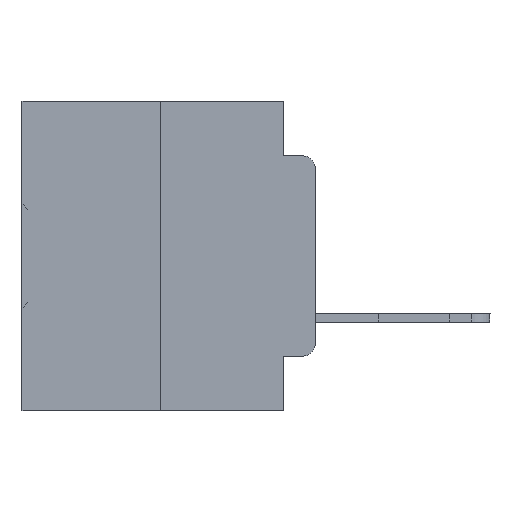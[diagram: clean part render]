
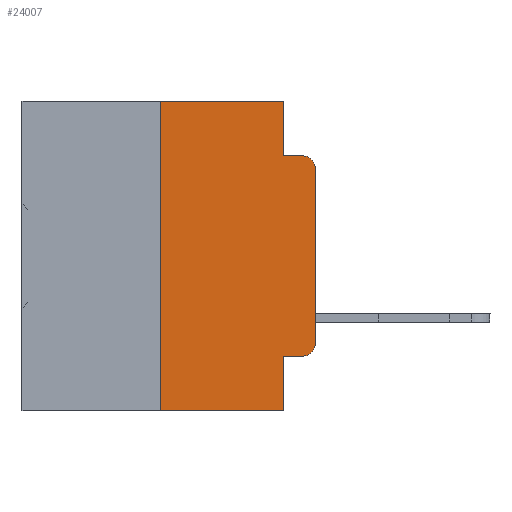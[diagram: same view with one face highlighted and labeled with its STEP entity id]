
A CAD part, left-side view. The second image highlights one B-rep face of the part: STEP entity #24007.
In plain terms, the highlighted planar face has unit normal (-1, 0, 0).
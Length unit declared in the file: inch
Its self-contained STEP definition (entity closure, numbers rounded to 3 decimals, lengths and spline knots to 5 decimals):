
#1431 = DIRECTION ( 'NONE',  ( 0., -1., 0. ) ) ;
#1639 = CARTESIAN_POINT ( 'NONE',  ( 0., 0.02, -0.3915 ) ) ;
#1751 = EDGE_CURVE ( 'NONE', #10572, #32576, #12706, .T. ) ;
#2280 = DIRECTION ( 'NONE',  ( 0., 0., -1. ) ) ;
#2330 = CARTESIAN_POINT ( 'NONE',  ( 0., 0.051, -0.0885 ) ) ;
#2474 = VERTEX_POINT ( 'NONE', #33356 ) ;
#2542 = VECTOR ( 'NONE', #15983, 39.37008 ) ;
#3257 = DIRECTION ( 'NONE',  ( 0., -1., 0. ) ) ;
#3674 = DIRECTION ( 'NONE',  ( -1., 0., 0. ) ) ;
#3776 = VECTOR ( 'NONE', #2280, 39.37008 ) ;
#4190 = LINE ( 'NONE', #15295, #14826 ) ;
#4243 = VERTEX_POINT ( 'NONE', #10545 ) ;
#4900 = VECTOR ( 'NONE', #3257, 39.37008 ) ;
#6938 = DIRECTION ( 'NONE',  ( 0., 0., -1. ) ) ;
#6973 = DIRECTION ( 'NONE',  ( 1., 0., 0. ) ) ;
#7317 = PLANE ( 'NONE',  #9222 ) ;
#7826 = CARTESIAN_POINT ( 'NONE',  ( 0., 0.25, 0. ) ) ;
#8423 = EDGE_CURVE ( 'NONE', #13669, #17629, #15838, .T. ) ;
#9222 = AXIS2_PLACEMENT_3D ( 'NONE', #9509, #6973, #15693 ) ;
#9509 = CARTESIAN_POINT ( 'NONE',  ( 0., 0.473, 0. ) ) ;
#9533 = CIRCLE ( 'NONE', #27577, 0.02 ) ;
#9961 = CARTESIAN_POINT ( 'NONE',  ( 0., 0.051, 0. ) ) ;
#10250 = LINE ( 'NONE', #35030, #19459 ) ;
#10407 = EDGE_CURVE ( 'NONE', #13234, #4243, #21440, .T. ) ;
#10545 = CARTESIAN_POINT ( 'NONE',  ( 0., 0.02, -0.4115 ) ) ;
#10572 = VERTEX_POINT ( 'NONE', #33083 ) ;
#11072 = CARTESIAN_POINT ( 'NONE',  ( 0., 0.473, -0.5 ) ) ;
#11238 = CIRCLE ( 'NONE', #25208, 0.02 ) ;
#11584 = CARTESIAN_POINT ( 'NONE',  ( 0., 0.473, 0. ) ) ;
#12706 = LINE ( 'NONE', #9961, #2542 ) ;
#13216 = VERTEX_POINT ( 'NONE', #15204 ) ;
#13234 = VERTEX_POINT ( 'NONE', #35925 ) ;
#13579 = CARTESIAN_POINT ( 'NONE',  ( 0., 0.02, -0.0885 ) ) ;
#13669 = VERTEX_POINT ( 'NONE', #21326 ) ;
#14146 = DIRECTION ( 'NONE',  ( 0., -1., 0. ) ) ;
#14826 = VECTOR ( 'NONE', #26382, 39.37008 ) ;
#15173 = FACE_OUTER_BOUND ( 'NONE', #26852, .T. ) ;
#15204 = CARTESIAN_POINT ( 'NONE',  ( 0., 0., -0.1085 ) ) ;
#15295 = CARTESIAN_POINT ( 'NONE',  ( 0., 0.051, -0.0885 ) ) ;
#15693 = DIRECTION ( 'NONE',  ( 0., 0., -1. ) ) ;
#15838 = LINE ( 'NONE', #7826, #35292 ) ;
#15983 = DIRECTION ( 'NONE',  ( 0., 0., -1. ) ) ;
#16492 = ORIENTED_EDGE ( 'NONE', *, *, #19468, .F. ) ;
#16832 = VERTEX_POINT ( 'NONE', #33874 ) ;
#17281 = CARTESIAN_POINT ( 'NONE',  ( 0., 0.02, -0.1085 ) ) ;
#17629 = VERTEX_POINT ( 'NONE', #31730 ) ;
#18929 = DIRECTION ( 'NONE',  ( 0., 0., 1. ) ) ;
#19459 = VECTOR ( 'NONE', #21204, 39.37008 ) ;
#19468 = EDGE_CURVE ( 'NONE', #32576, #22041, #4190, .T. ) ;
#19659 = DIRECTION ( 'NONE',  ( 0., 0., -1. ) ) ;
#20395 = ORIENTED_EDGE ( 'NONE', *, *, #1751, .F. ) ;
#20625 = VECTOR ( 'NONE', #14146, 39.37008 ) ;
#21204 = DIRECTION ( 'NONE',  ( 0., 0., 1. ) ) ;
#21292 = VECTOR ( 'NONE', #1431, 39.37008 ) ;
#21326 = CARTESIAN_POINT ( 'NONE',  ( 0., 0.25, -0.5 ) ) ;
#21388 = LINE ( 'NONE', #35399, #3776 ) ;
#21440 = LINE ( 'NONE', #27061, #21292 ) ;
#21472 = LINE ( 'NONE', #11072, #4900 ) ;
#22041 = VERTEX_POINT ( 'NONE', #13579 ) ;
#22885 = ORIENTED_EDGE ( 'NONE', *, *, #8423, .F. ) ;
#24007 = ADVANCED_FACE ( 'NONE', ( #15173 ), #7317, .F. ) ;
#24596 = EDGE_CURVE ( 'NONE', #13669, #2474, #21472, .T. ) ;
#25108 = DIRECTION ( 'NONE',  ( -1., 0., 0. ) ) ;
#25208 = AXIS2_PLACEMENT_3D ( 'NONE', #1639, #3674, #6938 ) ;
#25387 = EDGE_CURVE ( 'NONE', #16832, #13216, #10250, .T. ) ;
#25410 = EDGE_CURVE ( 'NONE', #13234, #2474, #21388, .T. ) ;
#25627 = ORIENTED_EDGE ( 'NONE', *, *, #10407, .T. ) ;
#25785 = ORIENTED_EDGE ( 'NONE', *, *, #24596, .T. ) ;
#26010 = ORIENTED_EDGE ( 'NONE', *, *, #25387, .T. ) ;
#26382 = DIRECTION ( 'NONE',  ( 0., -1., 0. ) ) ;
#26852 = EDGE_LOOP ( 'NONE', ( #26010, #33145, #16492, #20395, #35774, #22885, #25785, #33951, #25627, #31806 ) ) ;
#27061 = CARTESIAN_POINT ( 'NONE',  ( 0., 0.051, -0.4115 ) ) ;
#27577 = AXIS2_PLACEMENT_3D ( 'NONE', #17281, #25108, #19659 ) ;
#30534 = LINE ( 'NONE', #11584, #20625 ) ;
#30818 = EDGE_CURVE ( 'NONE', #4243, #16832, #11238, .T. ) ;
#31730 = CARTESIAN_POINT ( 'NONE',  ( 0., 0.25, 0. ) ) ;
#31806 = ORIENTED_EDGE ( 'NONE', *, *, #30818, .T. ) ;
#32341 = EDGE_CURVE ( 'NONE', #13216, #22041, #9533, .T. ) ;
#32576 = VERTEX_POINT ( 'NONE', #2330 ) ;
#32805 = EDGE_CURVE ( 'NONE', #17629, #10572, #30534, .T. ) ;
#33083 = CARTESIAN_POINT ( 'NONE',  ( 0., 0.051, 0. ) ) ;
#33145 = ORIENTED_EDGE ( 'NONE', *, *, #32341, .T. ) ;
#33356 = CARTESIAN_POINT ( 'NONE',  ( 0., 0.051, -0.5 ) ) ;
#33874 = CARTESIAN_POINT ( 'NONE',  ( 0., 0., -0.3915 ) ) ;
#33951 = ORIENTED_EDGE ( 'NONE', *, *, #25410, .F. ) ;
#35030 = CARTESIAN_POINT ( 'NONE',  ( 0., 0., 0. ) ) ;
#35292 = VECTOR ( 'NONE', #18929, 39.37008 ) ;
#35399 = CARTESIAN_POINT ( 'NONE',  ( 0., 0.051, 0. ) ) ;
#35774 = ORIENTED_EDGE ( 'NONE', *, *, #32805, .F. ) ;
#35925 = CARTESIAN_POINT ( 'NONE',  ( 0., 0.051, -0.4115 ) ) ;
